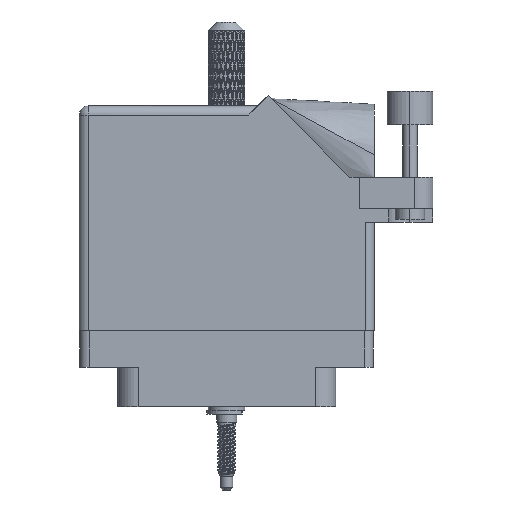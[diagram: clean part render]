
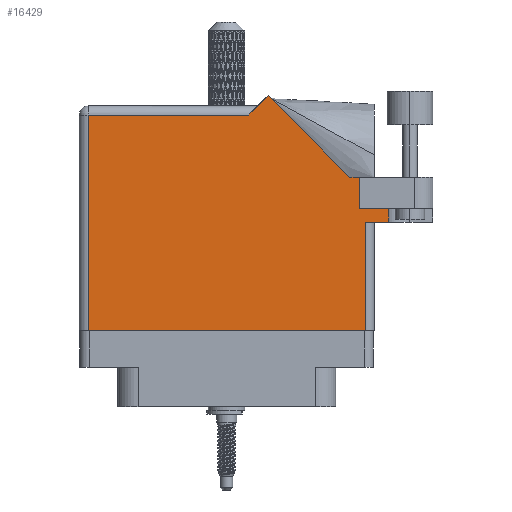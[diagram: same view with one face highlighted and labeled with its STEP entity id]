
A CAD part, front view. The second image highlights one B-rep face of the part: STEP entity #16429.
In plain terms, the highlighted face is planar.
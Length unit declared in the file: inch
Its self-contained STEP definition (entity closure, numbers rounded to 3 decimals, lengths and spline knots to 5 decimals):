
#2020 = DIRECTION ( 'NONE',  ( -0.707, 0.707, 0. ) ) ;
#2472 = DIRECTION ( 'NONE',  ( 1., 0., 0. ) ) ;
#4728 = VECTOR ( 'NONE', #2020, 39.37008 ) ;
#7678 = VERTEX_POINT ( 'NONE', #69851 ) ;
#10367 = VERTEX_POINT ( 'NONE', #65633 ) ;
#13724 = VERTEX_POINT ( 'NONE', #63886 ) ;
#14874 = EDGE_LOOP ( 'NONE', ( #94245, #53399, #25087, #67416, #62068, #72366, #72873, #52189, #85206, #42263, #34571 ) ) ;
#16429 = ADVANCED_FACE ( 'NONE', ( #100538 ), #77072, .F. ) ;
#19235 = VERTEX_POINT ( 'NONE', #86886 ) ;
#19362 = LINE ( 'NONE', #101203, #103989 ) ;
#24269 = EDGE_CURVE ( 'NONE', #19235, #13724, #70142, .T. ) ;
#25087 = ORIENTED_EDGE ( 'NONE', *, *, #25546, .T. ) ;
#25305 = CARTESIAN_POINT ( 'NONE',  ( -1.005, -0.1, 0.455 ) ) ;
#25546 = EDGE_CURVE ( 'NONE', #76246, #10367, #103328, .T. ) ;
#28337 = EDGE_CURVE ( 'NONE', #13724, #41233, #28663, .T. ) ;
#28663 = LINE ( 'NONE', #82369, #44139 ) ;
#31090 = AXIS2_PLACEMENT_3D ( 'NONE', #44785, #102160, #53028 ) ;
#31293 = CARTESIAN_POINT ( 'NONE',  ( 0.943, -0.1, 0.455 ) ) ;
#33264 = VERTEX_POINT ( 'NONE', #49583 ) ;
#33720 = DIRECTION ( 'NONE',  ( 1., 0., 0. ) ) ;
#34092 = VECTOR ( 'NONE', #71205, 39.37008 ) ;
#34571 = ORIENTED_EDGE ( 'NONE', *, *, #64255, .T. ) ;
#35917 = DIRECTION ( 'NONE',  ( 0., 1., 0. ) ) ;
#35984 = CARTESIAN_POINT ( 'NONE',  ( 1.005, 0.637, 0.455 ) ) ;
#39193 = LINE ( 'NONE', #103795, #34092 ) ;
#41233 = VERTEX_POINT ( 'NONE', #58006 ) ;
#42263 = ORIENTED_EDGE ( 'NONE', *, *, #63543, .T. ) ;
#42751 = VECTOR ( 'NONE', #2472, 39.37008 ) ;
#42865 = LINE ( 'NONE', #94286, #72375 ) ;
#43482 = DIRECTION ( 'NONE',  ( -1., 0., 0. ) ) ;
#44139 = VECTOR ( 'NONE', #89202, 39.37008 ) ;
#44778 = CARTESIAN_POINT ( 'NONE',  ( -0.943, 1.368, 0.455 ) ) ;
#44785 = CARTESIAN_POINT ( 'NONE',  ( -1.005, 1.43, 0.455 ) ) ;
#45599 = DIRECTION ( 'NONE',  ( -1., 0., 0. ) ) ;
#46326 = CARTESIAN_POINT ( 'NONE',  ( 0.905, 0.944, 0.455 ) ) ;
#48771 = CARTESIAN_POINT ( 'NONE',  ( 0.943, 0.637, 0.455 ) ) ;
#49583 = CARTESIAN_POINT ( 'NONE',  ( 0.905, 0.731, 0.455 ) ) ;
#50212 = EDGE_CURVE ( 'NONE', #33264, #57217, #42865, .T. ) ;
#51351 = DIRECTION ( 'NONE',  ( 1., 0., 0. ) ) ;
#52026 = VECTOR ( 'NONE', #51351, 39.37008 ) ;
#52189 = ORIENTED_EDGE ( 'NONE', *, *, #24269, .T. ) ;
#53028 = DIRECTION ( 'NONE',  ( -1., 0., 0. ) ) ;
#53399 = ORIENTED_EDGE ( 'NONE', *, *, #91047, .T. ) ;
#57217 = VERTEX_POINT ( 'NONE', #46326 ) ;
#58006 = CARTESIAN_POINT ( 'NONE',  ( 0.15, 1.368, 0.455 ) ) ;
#58319 = DIRECTION ( 'NONE',  ( 0., -1., 0. ) ) ;
#62068 = ORIENTED_EDGE ( 'NONE', *, *, #81012, .F. ) ;
#62685 = CARTESIAN_POINT ( 'NONE',  ( 1.1065, 1.06177, 0.455 ) ) ;
#63048 = DIRECTION ( 'NONE',  ( 0., -1., 0. ) ) ;
#63543 = EDGE_CURVE ( 'NONE', #41233, #71484, #74791, .T. ) ;
#63886 = CARTESIAN_POINT ( 'NONE',  ( 0.28271, 1.50071, 0.455 ) ) ;
#64255 = EDGE_CURVE ( 'NONE', #71484, #69276, #64575, .T. ) ;
#64350 = EDGE_CURVE ( 'NONE', #69276, #101316, #67165, .T. ) ;
#64575 = LINE ( 'NONE', #67315, #99211 ) ;
#65633 = CARTESIAN_POINT ( 'NONE',  ( 1.1065, 0.637, 0.455 ) ) ;
#67165 = LINE ( 'NONE', #25305, #42751 ) ;
#67315 = CARTESIAN_POINT ( 'NONE',  ( -0.943, -0.1, 0.455 ) ) ;
#67416 = ORIENTED_EDGE ( 'NONE', *, *, #82899, .F. ) ;
#67493 = CARTESIAN_POINT ( 'NONE',  ( -0.943, -0.1, 0.455 ) ) ;
#69276 = VERTEX_POINT ( 'NONE', #67493 ) ;
#69851 = CARTESIAN_POINT ( 'NONE',  ( 1.1065, 0.731, 0.455 ) ) ;
#70142 = LINE ( 'NONE', #84380, #4728 ) ;
#71205 = DIRECTION ( 'NONE',  ( 0., 1., 0. ) ) ;
#71484 = VERTEX_POINT ( 'NONE', #44778 ) ;
#72366 = ORIENTED_EDGE ( 'NONE', *, *, #50212, .T. ) ;
#72375 = VECTOR ( 'NONE', #35917, 39.37008 ) ;
#72873 = ORIENTED_EDGE ( 'NONE', *, *, #95531, .T. ) ;
#74791 = LINE ( 'NONE', #95768, #100432 ) ;
#76246 = VERTEX_POINT ( 'NONE', #48771 ) ;
#77072 = PLANE ( 'NONE',  #31090 ) ;
#78534 = VECTOR ( 'NONE', #33720, 39.37008 ) ;
#81012 = EDGE_CURVE ( 'NONE', #33264, #7678, #102912, .T. ) ;
#82369 = CARTESIAN_POINT ( 'NONE',  ( 0.212, 1.43, 0.455 ) ) ;
#82899 = EDGE_CURVE ( 'NONE', #7678, #10367, #87395, .T. ) ;
#84380 = CARTESIAN_POINT ( 'NONE',  ( 0.83942, 0.944, 0.455 ) ) ;
#85206 = ORIENTED_EDGE ( 'NONE', *, *, #28337, .T. ) ;
#86886 = CARTESIAN_POINT ( 'NONE',  ( 0.83942, 0.944, 0.455 ) ) ;
#87395 = LINE ( 'NONE', #62685, #104040 ) ;
#89202 = DIRECTION ( 'NONE',  ( -0.707, -0.707, 0. ) ) ;
#91047 = EDGE_CURVE ( 'NONE', #101316, #76246, #39193, .T. ) ;
#94245 = ORIENTED_EDGE ( 'NONE', *, *, #64350, .T. ) ;
#94286 = CARTESIAN_POINT ( 'NONE',  ( 0.905, 0.731, 0.455 ) ) ;
#95531 = EDGE_CURVE ( 'NONE', #57217, #19235, #19362, .T. ) ;
#95768 = CARTESIAN_POINT ( 'NONE',  ( -1.005, 1.368, 0.455 ) ) ;
#98222 = CARTESIAN_POINT ( 'NONE',  ( 0.905, 0.731, 0.455 ) ) ;
#99211 = VECTOR ( 'NONE', #58319, 39.37008 ) ;
#100432 = VECTOR ( 'NONE', #45599, 39.37008 ) ;
#100538 = FACE_OUTER_BOUND ( 'NONE', #14874, .T. ) ;
#101203 = CARTESIAN_POINT ( 'NONE',  ( 1.405, 0.944, 0.455 ) ) ;
#101316 = VERTEX_POINT ( 'NONE', #31293 ) ;
#102160 = DIRECTION ( 'NONE',  ( 0., 0., -1. ) ) ;
#102912 = LINE ( 'NONE', #98222, #78534 ) ;
#103328 = LINE ( 'NONE', #35984, #52026 ) ;
#103795 = CARTESIAN_POINT ( 'NONE',  ( 0.943, 0.637, 0.455 ) ) ;
#103989 = VECTOR ( 'NONE', #43482, 39.37008 ) ;
#104040 = VECTOR ( 'NONE', #63048, 39.37008 ) ;
